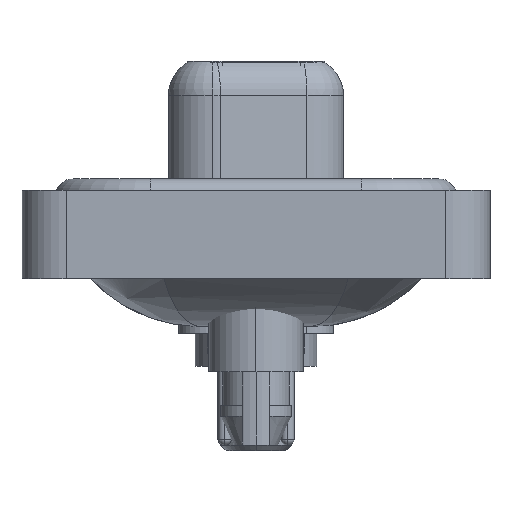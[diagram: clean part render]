
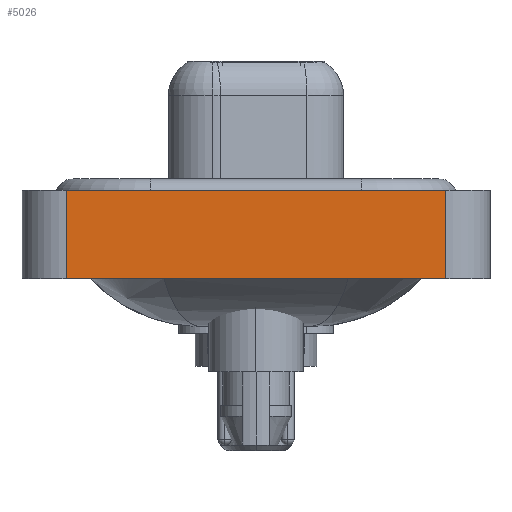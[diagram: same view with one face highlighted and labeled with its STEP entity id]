
A CAD part, left-side view. The second image highlights one B-rep face of the part: STEP entity #5026.
In plain terms, the highlighted planar face has unit normal (-1, 0, 0).
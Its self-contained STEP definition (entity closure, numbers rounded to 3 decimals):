
#330 = ORIENTED_EDGE ( 'NONE', *, *, #22957, .T. ) ;
#661 = LINE ( 'NONE', #6026, #19335 ) ;
#2297 = DIRECTION ( 'NONE',  ( 0., 0., 1. ) ) ;
#3341 = AXIS2_PLACEMENT_3D ( 'NONE', #7458, #12722, #18054 ) ;
#4237 = LINE ( 'NONE', #11366, #8217 ) ;
#4603 = CARTESIAN_POINT ( 'NONE',  ( -7.3, -8.55, -3.6 ) ) ;
#5026 = ADVANCED_FACE ( 'NONE', ( #18392 ), #16543, .T. ) ;
#5361 = DIRECTION ( 'NONE',  ( 0., -1., 0. ) ) ;
#5496 = ORIENTED_EDGE ( 'NONE', *, *, #9356, .F. ) ;
#6026 = CARTESIAN_POINT ( 'NONE',  ( -7.3, -8.55, -3.6 ) ) ;
#6044 = CARTESIAN_POINT ( 'NONE',  ( -7.3, 8.55, 0.4 ) ) ;
#7095 = EDGE_CURVE ( 'NONE', #18170, #14336, #22576, .T. ) ;
#7458 = CARTESIAN_POINT ( 'NONE',  ( -7.3, -8.55, -3.6 ) ) ;
#8217 = VECTOR ( 'NONE', #11474, 1000. ) ;
#8358 = ORIENTED_EDGE ( 'NONE', *, *, #7095, .F. ) ;
#8934 = EDGE_CURVE ( 'NONE', #20389, #15286, #661, .T. ) ;
#9356 = EDGE_CURVE ( 'NONE', #14336, #15286, #4237, .T. ) ;
#11011 = VECTOR ( 'NONE', #5361, 1000. ) ;
#11366 = CARTESIAN_POINT ( 'NONE',  ( -7.3, -8.55, 0.4 ) ) ;
#11474 = DIRECTION ( 'NONE',  ( 0., -1., 0. ) ) ;
#11818 = CARTESIAN_POINT ( 'NONE',  ( -7.3, -8.55, 0.4 ) ) ;
#12477 = ORIENTED_EDGE ( 'NONE', *, *, #8934, .T. ) ;
#12722 = DIRECTION ( 'NONE',  ( -1., 0., 0. ) ) ;
#13737 = CARTESIAN_POINT ( 'NONE',  ( -7.3, 8.55, -3.6 ) ) ;
#13780 = CARTESIAN_POINT ( 'NONE',  ( -7.3, 8.55, -3.6 ) ) ;
#14225 = LINE ( 'NONE', #21283, #11011 ) ;
#14336 = VERTEX_POINT ( 'NONE', #6044 ) ;
#15286 = VERTEX_POINT ( 'NONE', #11818 ) ;
#16543 = PLANE ( 'NONE',  #3341 ) ;
#18054 = DIRECTION ( 'NONE',  ( 0., 0., 1. ) ) ;
#18170 = VERTEX_POINT ( 'NONE', #13737 ) ;
#18392 = FACE_OUTER_BOUND ( 'NONE', #18805, .T. ) ;
#18695 = DIRECTION ( 'NONE',  ( 0., 0., 1. ) ) ;
#18805 = EDGE_LOOP ( 'NONE', ( #12477, #5496, #8358, #330 ) ) ;
#19335 = VECTOR ( 'NONE', #2297, 1000. ) ;
#20389 = VERTEX_POINT ( 'NONE', #4603 ) ;
#20729 = VECTOR ( 'NONE', #18695, 1000. ) ;
#21283 = CARTESIAN_POINT ( 'NONE',  ( -7.3, -8.55, -3.6 ) ) ;
#22576 = LINE ( 'NONE', #13780, #20729 ) ;
#22957 = EDGE_CURVE ( 'NONE', #18170, #20389, #14225, .T. ) ;
